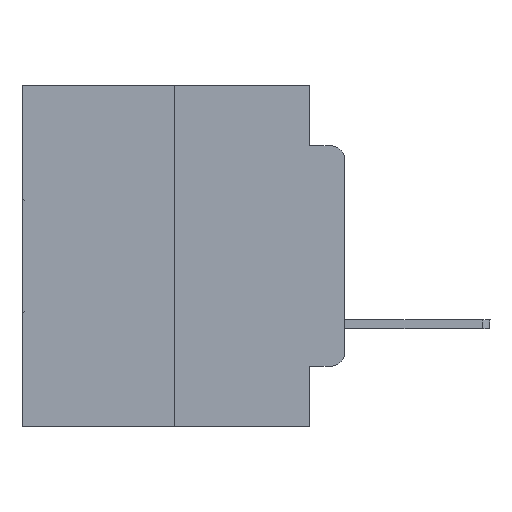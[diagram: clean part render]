
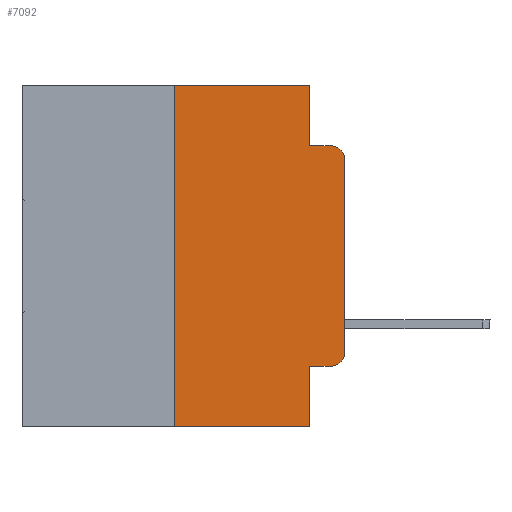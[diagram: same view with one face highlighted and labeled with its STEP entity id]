
A CAD part, left-side view. The second image highlights one B-rep face of the part: STEP entity #7092.
In plain terms, the highlighted planar face has unit normal (-1, 0, 0).
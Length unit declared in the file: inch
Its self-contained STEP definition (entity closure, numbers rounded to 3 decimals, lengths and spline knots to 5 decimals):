
#716 = CARTESIAN_POINT ( 'NONE',  ( 0., 0.051, -0.0885 ) ) ;
#917 = VECTOR ( 'NONE', #12659, 39.37008 ) ;
#1577 = EDGE_CURVE ( 'NONE', #10885, #24322, #16170, .T. ) ;
#1697 = VERTEX_POINT ( 'NONE', #25019 ) ;
#2040 = CARTESIAN_POINT ( 'NONE',  ( 0., 0., -0.3915 ) ) ;
#2384 = CARTESIAN_POINT ( 'NONE',  ( 0., 0.25, 0. ) ) ;
#2558 = DIRECTION ( 'NONE',  ( 0., 0., 1. ) ) ;
#2692 = LINE ( 'NONE', #12652, #5740 ) ;
#2739 = ORIENTED_EDGE ( 'NONE', *, *, #8373, .T. ) ;
#2865 = ORIENTED_EDGE ( 'NONE', *, *, #10815, .F. ) ;
#3175 = VERTEX_POINT ( 'NONE', #5265 ) ;
#3183 = DIRECTION ( 'NONE',  ( 1., 0., 0. ) ) ;
#4505 = CARTESIAN_POINT ( 'NONE',  ( 0., 0.02, -0.1085 ) ) ;
#4737 = CARTESIAN_POINT ( 'NONE',  ( 0., 0.051, -0.4115 ) ) ;
#5145 = LINE ( 'NONE', #716, #17824 ) ;
#5265 = CARTESIAN_POINT ( 'NONE',  ( 0., 0.051, -0.0885 ) ) ;
#5695 = VECTOR ( 'NONE', #2558, 39.37008 ) ;
#5740 = VECTOR ( 'NONE', #25352, 39.37008 ) ;
#5745 = CARTESIAN_POINT ( 'NONE',  ( 0., 0.051, 0. ) ) ;
#5831 = EDGE_CURVE ( 'NONE', #24322, #1697, #24462, .T. ) ;
#6007 = EDGE_CURVE ( 'NONE', #10885, #15821, #17287, .T. ) ;
#6479 = DIRECTION ( 'NONE',  ( 0., 0., -1. ) ) ;
#6559 = CARTESIAN_POINT ( 'NONE',  ( 0., 0., 0. ) ) ;
#7092 = ADVANCED_FACE ( 'NONE', ( #22174 ), #8094, .F. ) ;
#7452 = DIRECTION ( 'NONE',  ( 0., -1., 0. ) ) ;
#7781 = AXIS2_PLACEMENT_3D ( 'NONE', #4505, #13291, #19835 ) ;
#8018 = DIRECTION ( 'NONE',  ( 0., 0., -1. ) ) ;
#8094 = PLANE ( 'NONE',  #19797 ) ;
#8141 = EDGE_CURVE ( 'NONE', #20594, #11296, #9763, .T. ) ;
#8373 = EDGE_CURVE ( 'NONE', #11296, #12506, #27559, .T. ) ;
#8399 = VECTOR ( 'NONE', #16949, 39.37008 ) ;
#8683 = CARTESIAN_POINT ( 'NONE',  ( 0., 0.02, -0.4115 ) ) ;
#9763 = LINE ( 'NONE', #14880, #917 ) ;
#10077 = AXIS2_PLACEMENT_3D ( 'NONE', #21191, #23088, #8018 ) ;
#10306 = ORIENTED_EDGE ( 'NONE', *, *, #1577, .F. ) ;
#10626 = DIRECTION ( 'NONE',  ( 0., -1., 0. ) ) ;
#10815 = EDGE_CURVE ( 'NONE', #3175, #18303, #5145, .T. ) ;
#10885 = VERTEX_POINT ( 'NONE', #12605 ) ;
#11296 = VERTEX_POINT ( 'NONE', #8683 ) ;
#11508 = VERTEX_POINT ( 'NONE', #24850 ) ;
#12319 = EDGE_CURVE ( 'NONE', #20594, #15821, #23890, .T. ) ;
#12506 = VERTEX_POINT ( 'NONE', #2040 ) ;
#12605 = CARTESIAN_POINT ( 'NONE',  ( 0., 0.25, -0.5 ) ) ;
#12652 = CARTESIAN_POINT ( 'NONE',  ( 0., 0.051, 0. ) ) ;
#12659 = DIRECTION ( 'NONE',  ( 0., -1., 0. ) ) ;
#13291 = DIRECTION ( 'NONE',  ( -1., 0., 0. ) ) ;
#13319 = ORIENTED_EDGE ( 'NONE', *, *, #5831, .F. ) ;
#14206 = VECTOR ( 'NONE', #10626, 39.37008 ) ;
#14880 = CARTESIAN_POINT ( 'NONE',  ( 0., 0.051, -0.4115 ) ) ;
#15694 = VECTOR ( 'NONE', #27394, 39.37008 ) ;
#15821 = VERTEX_POINT ( 'NONE', #25665 ) ;
#15980 = LINE ( 'NONE', #6559, #5695 ) ;
#15999 = CIRCLE ( 'NONE', #7781, 0.02 ) ;
#16170 = LINE ( 'NONE', #22287, #16524 ) ;
#16524 = VECTOR ( 'NONE', #26661, 39.37008 ) ;
#16852 = CARTESIAN_POINT ( 'NONE',  ( 0., 0.473, 0. ) ) ;
#16949 = DIRECTION ( 'NONE',  ( 0., -1., 0. ) ) ;
#17287 = LINE ( 'NONE', #23721, #14206 ) ;
#17308 = ORIENTED_EDGE ( 'NONE', *, *, #18721, .T. ) ;
#17824 = VECTOR ( 'NONE', #7452, 39.37008 ) ;
#18303 = VERTEX_POINT ( 'NONE', #22784 ) ;
#18721 = EDGE_CURVE ( 'NONE', #12506, #11508, #15980, .T. ) ;
#19496 = ORIENTED_EDGE ( 'NONE', *, *, #19499, .F. ) ;
#19499 = EDGE_CURVE ( 'NONE', #1697, #3175, #2692, .T. ) ;
#19797 = AXIS2_PLACEMENT_3D ( 'NONE', #23305, #3183, #6479 ) ;
#19835 = DIRECTION ( 'NONE',  ( 0., 0., -1. ) ) ;
#19844 = EDGE_CURVE ( 'NONE', #11508, #18303, #15999, .T. ) ;
#20212 = ORIENTED_EDGE ( 'NONE', *, *, #12319, .F. ) ;
#20594 = VERTEX_POINT ( 'NONE', #4737 ) ;
#21191 = CARTESIAN_POINT ( 'NONE',  ( 0., 0.02, -0.3915 ) ) ;
#22174 = FACE_OUTER_BOUND ( 'NONE', #27673, .T. ) ;
#22287 = CARTESIAN_POINT ( 'NONE',  ( 0., 0.25, 0. ) ) ;
#22504 = ORIENTED_EDGE ( 'NONE', *, *, #8141, .T. ) ;
#22784 = CARTESIAN_POINT ( 'NONE',  ( 0., 0.02, -0.0885 ) ) ;
#22906 = ORIENTED_EDGE ( 'NONE', *, *, #19844, .T. ) ;
#23088 = DIRECTION ( 'NONE',  ( -1., 0., 0. ) ) ;
#23305 = CARTESIAN_POINT ( 'NONE',  ( 0., 0.473, 0. ) ) ;
#23721 = CARTESIAN_POINT ( 'NONE',  ( 0., 0.473, -0.5 ) ) ;
#23890 = LINE ( 'NONE', #5745, #15694 ) ;
#24322 = VERTEX_POINT ( 'NONE', #2384 ) ;
#24462 = LINE ( 'NONE', #16852, #8399 ) ;
#24850 = CARTESIAN_POINT ( 'NONE',  ( 0., 0., -0.1085 ) ) ;
#25019 = CARTESIAN_POINT ( 'NONE',  ( 0., 0.051, 0. ) ) ;
#25352 = DIRECTION ( 'NONE',  ( 0., 0., -1. ) ) ;
#25665 = CARTESIAN_POINT ( 'NONE',  ( 0., 0.051, -0.5 ) ) ;
#26661 = DIRECTION ( 'NONE',  ( 0., 0., 1. ) ) ;
#27394 = DIRECTION ( 'NONE',  ( 0., 0., -1. ) ) ;
#27559 = CIRCLE ( 'NONE', #10077, 0.02 ) ;
#27673 = EDGE_LOOP ( 'NONE', ( #17308, #22906, #2865, #19496, #13319, #10306, #27989, #20212, #22504, #2739 ) ) ;
#27989 = ORIENTED_EDGE ( 'NONE', *, *, #6007, .T. ) ;
